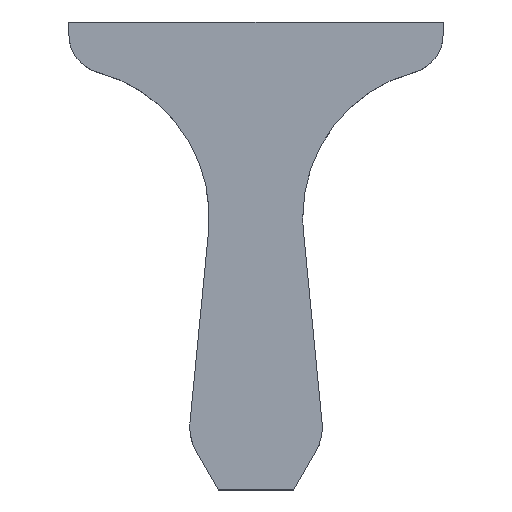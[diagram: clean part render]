
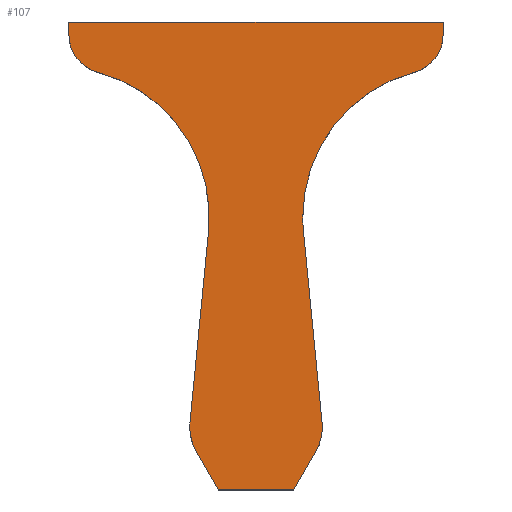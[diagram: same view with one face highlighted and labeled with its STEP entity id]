
A CAD part, top view. The second image highlights one B-rep face of the part: STEP entity #107.
In plain terms, the highlighted planar face has unit normal (0, 0, 1).
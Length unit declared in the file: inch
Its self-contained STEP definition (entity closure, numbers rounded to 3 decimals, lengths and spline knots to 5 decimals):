
#1 = VERTEX_POINT ( 'NONE', #321 ) ;
#3 = DIRECTION ( 'NONE',  ( 0., 0., 1. ) ) ;
#6 = DIRECTION ( 'NONE',  ( 0.5, -0.866, 0. ) ) ;
#8 = EDGE_CURVE ( 'NONE', #263, #458, #611, .T. ) ;
#17 = ORIENTED_EDGE ( 'NONE', *, *, #441, .T. ) ;
#35 = EDGE_CURVE ( 'NONE', #306, #49, #470, .T. ) ;
#37 = DIRECTION ( 'NONE',  ( 0., 0., -1. ) ) ;
#38 = DIRECTION ( 'NONE',  ( 1., 0., 0. ) ) ;
#42 = DIRECTION ( 'NONE',  ( -1., 0., 0. ) ) ;
#44 = CARTESIAN_POINT ( 'NONE',  ( -0.12, 0.25196, 0.03 ) ) ;
#49 = VERTEX_POINT ( 'NONE', #44 ) ;
#51 = AXIS2_PLACEMENT_3D ( 'NONE', #286, #622, #146 ) ;
#55 = DIRECTION ( 'NONE',  ( -0.097, 0.995, 0. ) ) ;
#56 = ORIENTED_EDGE ( 'NONE', *, *, #493, .T. ) ;
#64 = DIRECTION ( 'NONE',  ( 0., 0., 1. ) ) ;
#65 = EDGE_CURVE ( 'NONE', #442, #229, #274, .T. ) ;
#80 = CARTESIAN_POINT ( 'NONE',  ( -0.0242, -0.04, 0.03 ) ) ;
#81 = VECTOR ( 'NONE', #38, 39.37008 ) ;
#83 = CARTESIAN_POINT ( 'NONE',  ( 0.03, 0.135, 0.03 ) ) ;
#85 = CARTESIAN_POINT ( 'NONE',  ( 0.0115, 0., 0.03 ) ) ;
#96 = ORIENTED_EDGE ( 'NONE', *, *, #448, .T. ) ;
#107 = ADVANCED_FACE ( 'NONE', ( #204 ), #388, .T. ) ;
#116 = VECTOR ( 'NONE', #6, 39.37008 ) ;
#118 = AXIS2_PLACEMENT_3D ( 'NONE', #347, #287, #444 ) ;
#122 = ORIENTED_EDGE ( 'NONE', *, *, #503, .T. ) ;
#131 = DIRECTION ( 'NONE',  ( -0.097, -0.995, 0. ) ) ;
#142 = VERTEX_POINT ( 'NONE', #156 ) ;
#146 = DIRECTION ( 'NONE',  ( 1., 0., 0. ) ) ;
#154 = VECTOR ( 'NONE', #506, 39.37008 ) ;
#155 = CARTESIAN_POINT ( 'NONE',  ( -0.12, 0.26, 0.03 ) ) ;
#156 = CARTESIAN_POINT ( 'NONE',  ( -0.0425, 0., 0.03 ) ) ;
#160 = EDGE_CURVE ( 'NONE', #458, #142, #519, .T. ) ;
#165 = CARTESIAN_POINT ( 'NONE',  ( 0.0242, -0.04, 0.03 ) ) ;
#171 = VECTOR ( 'NONE', #603, 39.37008 ) ;
#173 = DIRECTION ( 'NONE',  ( 1., 0., 0. ) ) ;
#177 = DIRECTION ( 'NONE',  ( 0., 0., 1. ) ) ;
#179 = CIRCLE ( 'NONE', #621, 0.031 ) ;
#180 = DIRECTION ( 'NONE',  ( 0., 0., -1. ) ) ;
#183 = CARTESIAN_POINT ( 'NONE',  ( 0.12, 0.26, 0.03 ) ) ;
#186 = LINE ( 'NONE', #155, #619 ) ;
#195 = DIRECTION ( 'NONE',  ( 1., 0., 0. ) ) ;
#200 = EDGE_CURVE ( 'NONE', #245, #288, #526, .T. ) ;
#201 = CARTESIAN_POINT ( 'NONE',  ( -0.03835, -0.0155, 0.03 ) ) ;
#203 = EDGE_CURVE ( 'NONE', #142, #280, #179, .T. ) ;
#204 = FACE_OUTER_BOUND ( 'NONE', #612, .T. ) ;
#205 = CARTESIAN_POINT ( 'NONE',  ( 0.095, 0.25196, 0.03 ) ) ;
#207 = AXIS2_PLACEMENT_3D ( 'NONE', #85, #364, #42 ) ;
#210 = ORIENTED_EDGE ( 'NONE', *, *, #476, .T. ) ;
#215 = ORIENTED_EDGE ( 'NONE', *, *, #528, .T. ) ;
#217 = CARTESIAN_POINT ( 'NONE',  ( -0.03045, 0.12573, 0.03 ) ) ;
#220 = LINE ( 'NONE', #273, #268 ) ;
#222 = ORIENTED_EDGE ( 'NONE', *, *, #35, .T. ) ;
#224 = DIRECTION ( 'NONE',  ( -1., 0., 0. ) ) ;
#229 = VERTEX_POINT ( 'NONE', #165 ) ;
#230 = CARTESIAN_POINT ( 'NONE',  ( -0.04236, 0.00299, 0.03 ) ) ;
#232 = VERTEX_POINT ( 'NONE', #405 ) ;
#239 = CARTESIAN_POINT ( 'NONE',  ( -0.0115, 0., 0.03 ) ) ;
#245 = VERTEX_POINT ( 'NONE', #254 ) ;
#253 = DIRECTION ( 'NONE',  ( 1., 0., 0. ) ) ;
#254 = CARTESIAN_POINT ( 'NONE',  ( 0.04236, 0.00299, 0.03 ) ) ;
#263 = VERTEX_POINT ( 'NONE', #217 ) ;
#268 = VECTOR ( 'NONE', #269, 39.37008 ) ;
#269 = DIRECTION ( 'NONE',  ( 0.5, 0.866, 0. ) ) ;
#273 = CARTESIAN_POINT ( 'NONE',  ( 0.03835, -0.0155, 0.03 ) ) ;
#274 = LINE ( 'NONE', #80, #81 ) ;
#280 = VERTEX_POINT ( 'NONE', #361 ) ;
#281 = CARTESIAN_POINT ( 'NONE',  ( -0.095, 0.25196, 0.03 ) ) ;
#282 = ORIENTED_EDGE ( 'NONE', *, *, #160, .T. ) ;
#284 = VERTEX_POINT ( 'NONE', #307 ) ;
#285 = EDGE_CURVE ( 'NONE', #598, #284, #352, .T. ) ;
#286 = CARTESIAN_POINT ( 'NONE',  ( 0.126, 0.135, 0.03 ) ) ;
#287 = DIRECTION ( 'NONE',  ( 0., 0., 1. ) ) ;
#288 = VERTEX_POINT ( 'NONE', #500 ) ;
#292 = VECTOR ( 'NONE', #55, 39.37008 ) ;
#297 = LINE ( 'NONE', #201, #116 ) ;
#306 = VERTEX_POINT ( 'NONE', #350 ) ;
#307 = CARTESIAN_POINT ( 'NONE',  ( 0.12, 0.25196, 0.03 ) ) ;
#315 = CARTESIAN_POINT ( 'NONE',  ( -0.0242, -0.04, 0.03 ) ) ;
#318 = AXIS2_PLACEMENT_3D ( 'NONE', #427, #37, #224 ) ;
#321 = CARTESIAN_POINT ( 'NONE',  ( 0.12, 0.26, 0.03 ) ) ;
#330 = CIRCLE ( 'NONE', #207, 0.031 ) ;
#332 = ORIENTED_EDGE ( 'NONE', *, *, #417, .T. ) ;
#339 = CARTESIAN_POINT ( 'NONE',  ( 0.03045, 0.12573, 0.03 ) ) ;
#347 = CARTESIAN_POINT ( 'NONE',  ( -0.095, 0.25196, 0.03 ) ) ;
#350 = CARTESIAN_POINT ( 'NONE',  ( -0.12, 0.26, 0.03 ) ) ;
#352 = CIRCLE ( 'NONE', #573, 0.025 ) ;
#360 = AXIS2_PLACEMENT_3D ( 'NONE', #239, #64, #253 ) ;
#361 = CARTESIAN_POINT ( 'NONE',  ( -0.03835, -0.0155, 0.03 ) ) ;
#364 = DIRECTION ( 'NONE',  ( 0., 0., 1. ) ) ;
#368 = AXIS2_PLACEMENT_3D ( 'NONE', #281, #177, #565 ) ;
#375 = ORIENTED_EDGE ( 'NONE', *, *, #200, .T. ) ;
#378 = EDGE_CURVE ( 'NONE', #284, #1, #556, .T. ) ;
#386 = ORIENTED_EDGE ( 'NONE', *, *, #378, .T. ) ;
#388 = PLANE ( 'NONE',  #118 ) ;
#395 = CIRCLE ( 'NONE', #318, 0.096 ) ;
#397 = VECTOR ( 'NONE', #131, 39.37008 ) ;
#402 = DIRECTION ( 'NONE',  ( 0., 0., 1. ) ) ;
#405 = CARTESIAN_POINT ( 'NONE',  ( 0.03835, -0.0155, 0.03 ) ) ;
#417 = EDGE_CURVE ( 'NONE', #49, #572, #551, .T. ) ;
#423 = ORIENTED_EDGE ( 'NONE', *, *, #8, .T. ) ;
#427 = CARTESIAN_POINT ( 'NONE',  ( -0.126, 0.135, 0.03 ) ) ;
#432 = VERTEX_POINT ( 'NONE', #83 ) ;
#434 = ORIENTED_EDGE ( 'NONE', *, *, #464, .T. ) ;
#440 = CARTESIAN_POINT ( 'NONE',  ( -0.0115, 0., 0.03 ) ) ;
#441 = EDGE_CURVE ( 'NONE', #432, #598, #608, .T. ) ;
#442 = VERTEX_POINT ( 'NONE', #315 ) ;
#444 = DIRECTION ( 'NONE',  ( 1., 0., 0. ) ) ;
#448 = EDGE_CURVE ( 'NONE', #232, #245, #330, .T. ) ;
#453 = ORIENTED_EDGE ( 'NONE', *, *, #65, .T. ) ;
#454 = AXIS2_PLACEMENT_3D ( 'NONE', #478, #180, #173 ) ;
#458 = VERTEX_POINT ( 'NONE', #230 ) ;
#464 = EDGE_CURVE ( 'NONE', #229, #232, #220, .T. ) ;
#470 = LINE ( 'NONE', #576, #154 ) ;
#476 = EDGE_CURVE ( 'NONE', #572, #263, #395, .T. ) ;
#478 = CARTESIAN_POINT ( 'NONE',  ( 0.126, 0.135, 0.03 ) ) ;
#479 = ORIENTED_EDGE ( 'NONE', *, *, #285, .T. ) ;
#484 = DIRECTION ( 'NONE',  ( -1., 0., 0. ) ) ;
#493 = EDGE_CURVE ( 'NONE', #280, #442, #297, .T. ) ;
#500 = CARTESIAN_POINT ( 'NONE',  ( 0.03045, 0.12573, 0.03 ) ) ;
#503 = EDGE_CURVE ( 'NONE', #1, #306, #186, .T. ) ;
#506 = DIRECTION ( 'NONE',  ( 0., -1., 0. ) ) ;
#519 = CIRCLE ( 'NONE', #360, 0.031 ) ;
#526 = LINE ( 'NONE', #339, #292 ) ;
#527 = ORIENTED_EDGE ( 'NONE', *, *, #203, .T. ) ;
#528 = EDGE_CURVE ( 'NONE', #288, #432, #548, .T. ) ;
#532 = CARTESIAN_POINT ( 'NONE',  ( 0.1014, 0.2278, 0.03 ) ) ;
#548 = CIRCLE ( 'NONE', #51, 0.096 ) ;
#551 = CIRCLE ( 'NONE', #368, 0.025 ) ;
#552 = DIRECTION ( 'NONE',  ( -1., 0., 0. ) ) ;
#556 = LINE ( 'NONE', #183, #171 ) ;
#563 = CARTESIAN_POINT ( 'NONE',  ( -0.03045, 0.12573, 0.03 ) ) ;
#565 = DIRECTION ( 'NONE',  ( 1., 0., 0. ) ) ;
#572 = VERTEX_POINT ( 'NONE', #574 ) ;
#573 = AXIS2_PLACEMENT_3D ( 'NONE', #205, #402, #552 ) ;
#574 = CARTESIAN_POINT ( 'NONE',  ( -0.1014, 0.2278, 0.03 ) ) ;
#576 = CARTESIAN_POINT ( 'NONE',  ( -0.12, 0.26, 0.03 ) ) ;
#598 = VERTEX_POINT ( 'NONE', #532 ) ;
#603 = DIRECTION ( 'NONE',  ( 0., 1., 0. ) ) ;
#608 = CIRCLE ( 'NONE', #454, 0.096 ) ;
#611 = LINE ( 'NONE', #563, #397 ) ;
#612 = EDGE_LOOP ( 'NONE', ( #222, #332, #210, #423, #282, #527, #56, #453, #434, #96, #375, #215, #17, #479, #386, #122 ) ) ;
#619 = VECTOR ( 'NONE', #484, 39.37008 ) ;
#621 = AXIS2_PLACEMENT_3D ( 'NONE', #440, #3, #195 ) ;
#622 = DIRECTION ( 'NONE',  ( 0., 0., -1. ) ) ;
